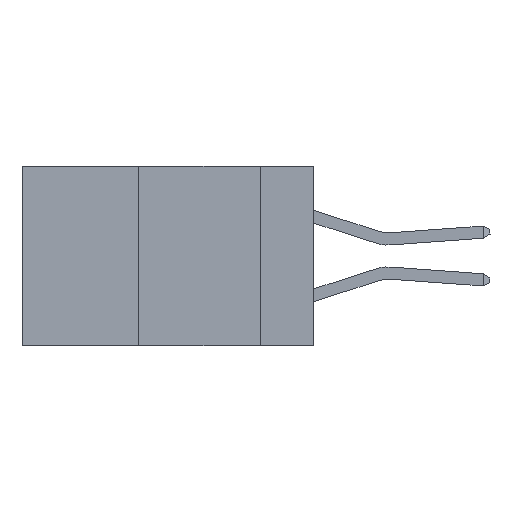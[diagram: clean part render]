
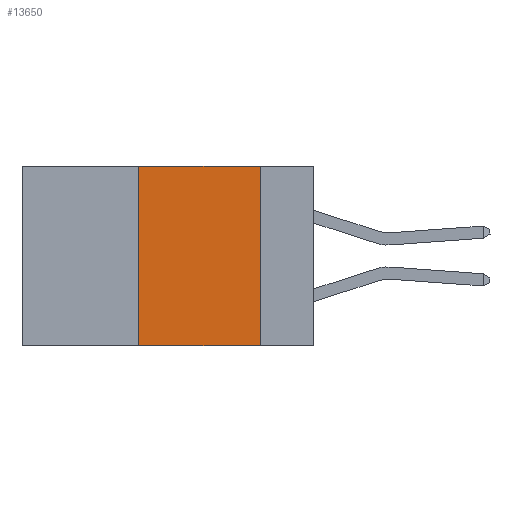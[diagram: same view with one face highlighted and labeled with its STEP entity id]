
A CAD part, left-side view. The second image highlights one B-rep face of the part: STEP entity #13650.
In plain terms, the highlighted planar face has unit normal (-1, 0, 0).
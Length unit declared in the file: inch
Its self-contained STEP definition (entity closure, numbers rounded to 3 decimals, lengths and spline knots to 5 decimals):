
#31 = CARTESIAN_POINT ( 'NONE',  ( 0., 0.11, 0. ) ) ;
#509 = VERTEX_POINT ( 'NONE', #10868 ) ;
#644 = LINE ( 'NONE', #3921, #13600 ) ;
#773 = VECTOR ( 'NONE', #3150, 39.37008 ) ;
#780 = VECTOR ( 'NONE', #12107, 39.37008 ) ;
#873 = EDGE_CURVE ( 'NONE', #509, #10486, #10638, .T. ) ;
#946 = DIRECTION ( 'NONE',  ( 1., 0., 0. ) ) ;
#1066 = VERTEX_POINT ( 'NONE', #8917 ) ;
#1152 = ORIENTED_EDGE ( 'NONE', *, *, #2560, .F. ) ;
#1552 = DIRECTION ( 'NONE',  ( 0., 0., 1. ) ) ;
#2031 = ORIENTED_EDGE ( 'NONE', *, *, #3451, .F. ) ;
#2560 = EDGE_CURVE ( 'NONE', #10486, #1066, #644, .T. ) ;
#3120 = EDGE_LOOP ( 'NONE', ( #1152, #12574, #2031, #13978 ) ) ;
#3150 = DIRECTION ( 'NONE',  ( 0., -1., 0. ) ) ;
#3451 = EDGE_CURVE ( 'NONE', #6662, #509, #6945, .T. ) ;
#3818 = CARTESIAN_POINT ( 'NONE',  ( 0., 0.36, 0. ) ) ;
#3921 = CARTESIAN_POINT ( 'NONE',  ( 0., 0.11, 0. ) ) ;
#4675 = CARTESIAN_POINT ( 'NONE',  ( 0., 0.36, -0.37 ) ) ;
#6211 = PLANE ( 'NONE',  #12404 ) ;
#6274 = VECTOR ( 'NONE', #1552, 39.37008 ) ;
#6662 = VERTEX_POINT ( 'NONE', #4675 ) ;
#6945 = LINE ( 'NONE', #3818, #6274 ) ;
#6979 = DIRECTION ( 'NONE',  ( 0., 0., -1. ) ) ;
#7345 = CARTESIAN_POINT ( 'NONE',  ( 0., 0.6, 0. ) ) ;
#7421 = FACE_OUTER_BOUND ( 'NONE', #3120, .T. ) ;
#8347 = CARTESIAN_POINT ( 'NONE',  ( 0., 0.6, 0. ) ) ;
#8768 = LINE ( 'NONE', #9763, #780 ) ;
#8917 = CARTESIAN_POINT ( 'NONE',  ( 0., 0.11, -0.37 ) ) ;
#9641 = DIRECTION ( 'NONE',  ( 0., 0., -1. ) ) ;
#9763 = CARTESIAN_POINT ( 'NONE',  ( 0., 0.6, -0.37 ) ) ;
#10486 = VERTEX_POINT ( 'NONE', #31 ) ;
#10638 = LINE ( 'NONE', #8347, #773 ) ;
#10868 = CARTESIAN_POINT ( 'NONE',  ( 0., 0.36, 0. ) ) ;
#12107 = DIRECTION ( 'NONE',  ( 0., -1., 0. ) ) ;
#12404 = AXIS2_PLACEMENT_3D ( 'NONE', #7345, #946, #9641 ) ;
#12574 = ORIENTED_EDGE ( 'NONE', *, *, #873, .F. ) ;
#12957 = EDGE_CURVE ( 'NONE', #6662, #1066, #8768, .T. ) ;
#13600 = VECTOR ( 'NONE', #6979, 39.37008 ) ;
#13650 = ADVANCED_FACE ( 'NONE', ( #7421 ), #6211, .F. ) ;
#13978 = ORIENTED_EDGE ( 'NONE', *, *, #12957, .T. ) ;
